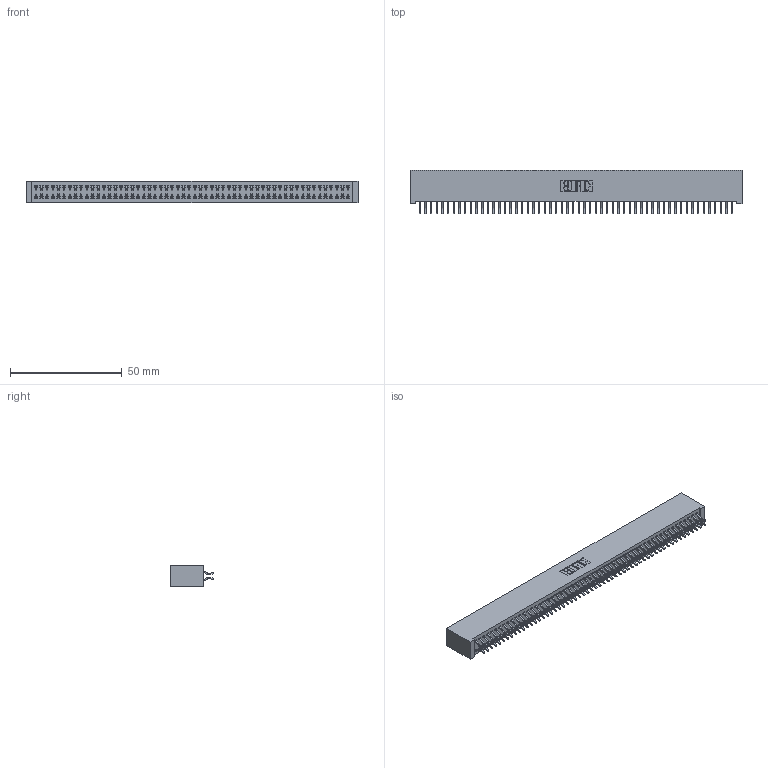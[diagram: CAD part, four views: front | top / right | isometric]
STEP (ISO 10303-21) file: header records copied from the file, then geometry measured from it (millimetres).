
FILE_DESCRIPTION (( 'STEP AP203' ), '1' );
FILE_NAME ('342-112-556-201.STEP', '2018-08-14T12:24:37', ( '' ), ( '' ), 'SwSTEP 2.0', 'SolidWorks 2016', '' );
FILE_SCHEMA (( 'CONFIG_CONTROL_DESIGN' ));
Length unit declared in the file: inch
Products named in the file (3): 342 Part_Lugless; 345-292-001_556 Tail; 342-112-556-201
Assembly tree (113 placements, depth 2):
  342-112-556-201
    342 Part_Lugless
    345-292-001_556 Tail  x112
Bounding box: 148.49 x 19.58 x 9.4 mm (x, y, z)
Volume: 13844.6 mm3; surface area: 23218.1 mm2
Topology: 113 solids, 113 shells, 6598 faces, 19651 edges, 12950 vertices
Faces by surface type: plane 4542, cylinder 2056
Entity records: 34027 total; most frequent: CARTESIAN_POINT 5634, ORIENTED_EDGE 5558, DIRECTION 4771, EDGE_CURVE 2779, LINE 2651, VECTOR 2651, VERTEX_POINT 1850, AXIS2_PLACEMENT_3D 1060
